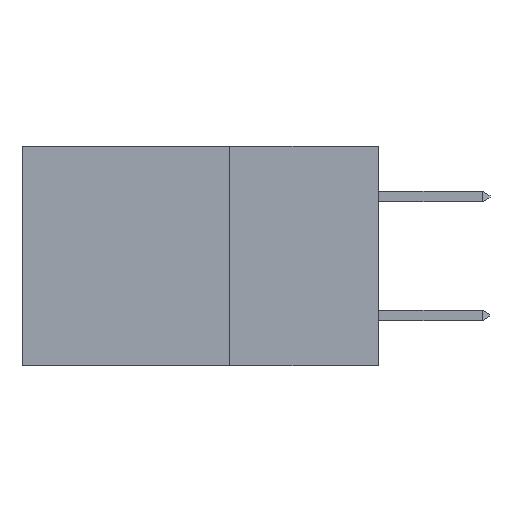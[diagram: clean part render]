
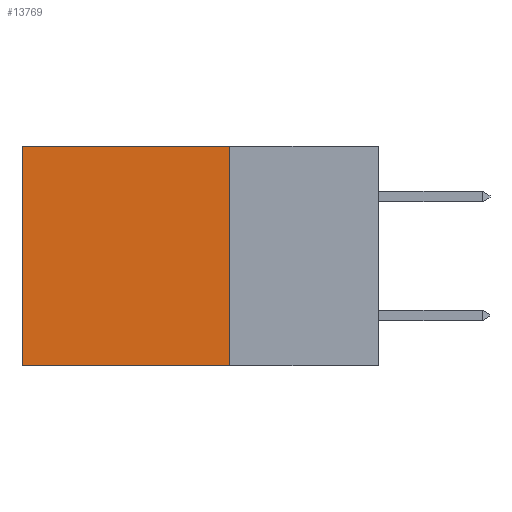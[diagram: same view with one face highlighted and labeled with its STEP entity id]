
A CAD part, left-side view. The second image highlights one B-rep face of the part: STEP entity #13769.
In plain terms, the highlighted planar face has unit normal (-1, 0, 0).
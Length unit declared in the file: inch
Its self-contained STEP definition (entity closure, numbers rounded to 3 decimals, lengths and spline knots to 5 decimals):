
#122 = DIRECTION ( 'NONE',  ( 0., 0., -1. ) ) ;
#452 = EDGE_CURVE ( 'NONE', #9639, #16316, #8543, .T. ) ;
#1610 = DIRECTION ( 'NONE',  ( 0., 0., -1. ) ) ;
#2632 = VERTEX_POINT ( 'NONE', #13120 ) ;
#2791 = EDGE_LOOP ( 'NONE', ( #13948, #5862, #13294, #3596 ) ) ;
#3596 = ORIENTED_EDGE ( 'NONE', *, *, #7212, .T. ) ;
#4913 = FACE_OUTER_BOUND ( 'NONE', #2791, .T. ) ;
#5755 = VERTEX_POINT ( 'NONE', #13323 ) ;
#5862 = ORIENTED_EDGE ( 'NONE', *, *, #12057, .F. ) ;
#6579 = VECTOR ( 'NONE', #7635, 39.37008 ) ;
#6937 = LINE ( 'NONE', #10537, #17059 ) ;
#7212 = EDGE_CURVE ( 'NONE', #5755, #9639, #6937, .T. ) ;
#7635 = DIRECTION ( 'NONE',  ( 0., 1., 0. ) ) ;
#8131 = VECTOR ( 'NONE', #1610, 39.37008 ) ;
#8146 = DIRECTION ( 'NONE',  ( 1., 0., 0. ) ) ;
#8530 = CARTESIAN_POINT ( 'NONE',  ( 0.298, 0.6, 0. ) ) ;
#8543 = LINE ( 'NONE', #8530, #8131 ) ;
#9275 = CARTESIAN_POINT ( 'NONE',  ( 0.298, 0.6, 0. ) ) ;
#9639 = VERTEX_POINT ( 'NONE', #9275 ) ;
#10482 = DIRECTION ( 'NONE',  ( 0., 1., 0. ) ) ;
#10537 = CARTESIAN_POINT ( 'NONE',  ( 0.298, 0.25, 0. ) ) ;
#11883 = CARTESIAN_POINT ( 'NONE',  ( 0.298, 0.6, -0.37 ) ) ;
#12057 = EDGE_CURVE ( 'NONE', #2632, #16316, #13586, .T. ) ;
#13120 = CARTESIAN_POINT ( 'NONE',  ( 0.298, 0.25, -0.37 ) ) ;
#13294 = ORIENTED_EDGE ( 'NONE', *, *, #14598, .F. ) ;
#13323 = CARTESIAN_POINT ( 'NONE',  ( 0.298, 0.25, 0. ) ) ;
#13384 = PLANE ( 'NONE',  #15903 ) ;
#13468 = LINE ( 'NONE', #14995, #16590 ) ;
#13586 = LINE ( 'NONE', #16849, #6579 ) ;
#13769 = ADVANCED_FACE ( 'NONE', ( #4913 ), #13384, .F. ) ;
#13948 = ORIENTED_EDGE ( 'NONE', *, *, #452, .T. ) ;
#14598 = EDGE_CURVE ( 'NONE', #5755, #2632, #13468, .T. ) ;
#14995 = CARTESIAN_POINT ( 'NONE',  ( 0.298, 0.25, 0. ) ) ;
#15903 = AXIS2_PLACEMENT_3D ( 'NONE', #16077, #8146, #122 ) ;
#16077 = CARTESIAN_POINT ( 'NONE',  ( 0.298, 0.25, 0. ) ) ;
#16316 = VERTEX_POINT ( 'NONE', #11883 ) ;
#16336 = DIRECTION ( 'NONE',  ( 0., 0., -1. ) ) ;
#16590 = VECTOR ( 'NONE', #16336, 39.37008 ) ;
#16849 = CARTESIAN_POINT ( 'NONE',  ( 0.298, 0.25, -0.37 ) ) ;
#17059 = VECTOR ( 'NONE', #10482, 39.37008 ) ;
